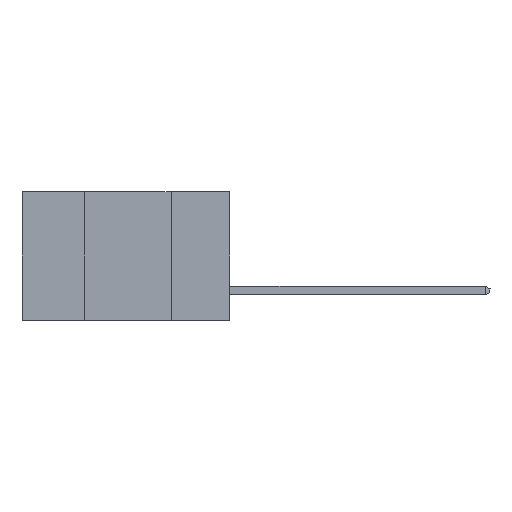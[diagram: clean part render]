
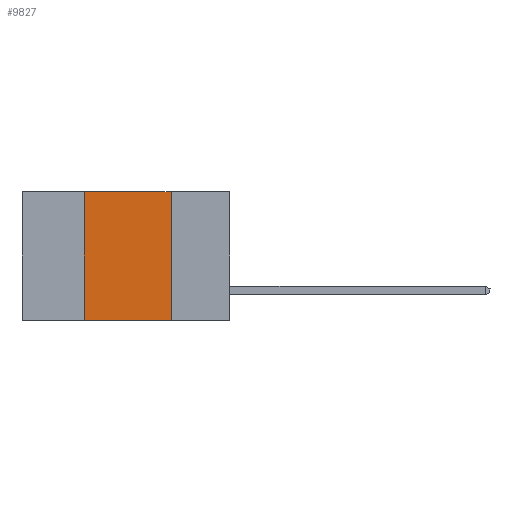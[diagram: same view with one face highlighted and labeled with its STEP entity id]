
A CAD part, left-side view. The second image highlights one B-rep face of the part: STEP entity #9827.
In plain terms, the highlighted planar face has unit normal (-1, 0, 0).
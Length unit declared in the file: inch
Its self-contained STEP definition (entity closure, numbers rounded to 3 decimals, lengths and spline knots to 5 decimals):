
#270 = CARTESIAN_POINT ( 'NONE',  ( 0., 0.6, -0.37 ) ) ;
#325 = DIRECTION ( 'NONE',  ( 0., -1., 0. ) ) ;
#406 = ORIENTED_EDGE ( 'NONE', *, *, #3420, .F. ) ;
#497 = DIRECTION ( 'NONE',  ( 0., 0., -1. ) ) ;
#519 = PLANE ( 'NONE',  #1154 ) ;
#705 = DIRECTION ( 'NONE',  ( 0., 0., 1. ) ) ;
#1124 = FACE_OUTER_BOUND ( 'NONE', #6126, .T. ) ;
#1154 = AXIS2_PLACEMENT_3D ( 'NONE', #9584, #5742, #7455 ) ;
#1223 = LINE ( 'NONE', #4229, #3870 ) ;
#1735 = CARTESIAN_POINT ( 'NONE',  ( 0., 0.17, -0.37 ) ) ;
#1978 = CARTESIAN_POINT ( 'NONE',  ( 0., 0.42, 0. ) ) ;
#2388 = VERTEX_POINT ( 'NONE', #3493 ) ;
#2875 = CARTESIAN_POINT ( 'NONE',  ( 0., 0.42, -0.37 ) ) ;
#3242 = VERTEX_POINT ( 'NONE', #1978 ) ;
#3397 = CARTESIAN_POINT ( 'NONE',  ( 0., 0.17, 0. ) ) ;
#3420 = EDGE_CURVE ( 'NONE', #2388, #3242, #7582, .T. ) ;
#3493 = CARTESIAN_POINT ( 'NONE',  ( 0., 0.42, -0.37 ) ) ;
#3519 = VECTOR ( 'NONE', #325, 39.37008 ) ;
#3870 = VECTOR ( 'NONE', #8071, 39.37008 ) ;
#4057 = VERTEX_POINT ( 'NONE', #1735 ) ;
#4091 = LINE ( 'NONE', #270, #3519 ) ;
#4229 = CARTESIAN_POINT ( 'NONE',  ( 0., 0.6, 0. ) ) ;
#4258 = LINE ( 'NONE', #5972, #4778 ) ;
#4778 = VECTOR ( 'NONE', #497, 39.37008 ) ;
#5351 = ORIENTED_EDGE ( 'NONE', *, *, #9451, .F. ) ;
#5440 = EDGE_CURVE ( 'NONE', #2388, #4057, #4091, .T. ) ;
#5505 = VERTEX_POINT ( 'NONE', #3397 ) ;
#5589 = EDGE_CURVE ( 'NONE', #5505, #4057, #4258, .T. ) ;
#5742 = DIRECTION ( 'NONE',  ( 1., 0., 0. ) ) ;
#5972 = CARTESIAN_POINT ( 'NONE',  ( 0., 0.17, -0.37 ) ) ;
#6126 = EDGE_LOOP ( 'NONE', ( #8122, #5351, #406, #7063 ) ) ;
#7063 = ORIENTED_EDGE ( 'NONE', *, *, #5440, .T. ) ;
#7455 = DIRECTION ( 'NONE',  ( 0., 0., -1. ) ) ;
#7582 = LINE ( 'NONE', #2875, #7657 ) ;
#7657 = VECTOR ( 'NONE', #705, 39.37008 ) ;
#8071 = DIRECTION ( 'NONE',  ( 0., -1., 0. ) ) ;
#8122 = ORIENTED_EDGE ( 'NONE', *, *, #5589, .F. ) ;
#9451 = EDGE_CURVE ( 'NONE', #3242, #5505, #1223, .T. ) ;
#9584 = CARTESIAN_POINT ( 'NONE',  ( 0., 0.6, 0. ) ) ;
#9827 = ADVANCED_FACE ( 'NONE', ( #1124 ), #519, .F. ) ;
